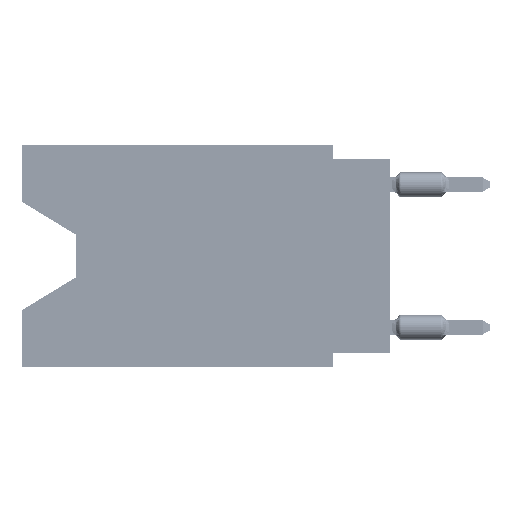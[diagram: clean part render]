
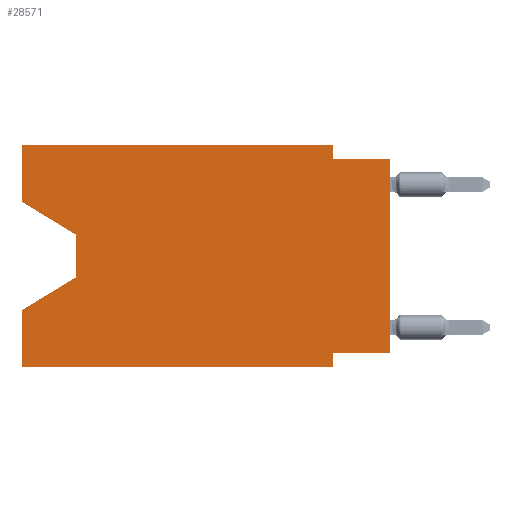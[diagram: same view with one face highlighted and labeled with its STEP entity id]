
A CAD part, left-side view. The second image highlights one B-rep face of the part: STEP entity #28571.
In plain terms, the highlighted planar face has unit normal (-1, 0, 0).
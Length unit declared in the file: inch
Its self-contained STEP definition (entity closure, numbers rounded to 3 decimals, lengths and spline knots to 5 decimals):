
#1226 = ORIENTED_EDGE ( 'NONE', *, *, #63937, .T. ) ;
#1732 = VERTEX_POINT ( 'NONE', #47006 ) ;
#1911 = AXIS2_PLACEMENT_3D ( 'NONE', #13726, #6431, #18738 ) ;
#3129 = ORIENTED_EDGE ( 'NONE', *, *, #56652, .T. ) ;
#3431 = DIRECTION ( 'NONE',  ( 0., 0., 1. ) ) ;
#3860 = VECTOR ( 'NONE', #61760, 39.37008 ) ;
#3981 = EDGE_CURVE ( 'NONE', #13742, #73121, #71780, .T. ) ;
#4955 = EDGE_LOOP ( 'NONE', ( #50636, #10048, #3129, #48341, #44960, #50207, #41376, #1226, #11884, #43274, #49702, #40008 ) ) ;
#5191 = LINE ( 'NONE', #29465, #14476 ) ;
#5551 = CARTESIAN_POINT ( 'NONE',  ( 0., 0., -0.025 ) ) ;
#6381 = VERTEX_POINT ( 'NONE', #11657 ) ;
#6431 = DIRECTION ( 'NONE',  ( 1., 0., 0. ) ) ;
#7757 = VECTOR ( 'NONE', #19069, 39.37008 ) ;
#9635 = VECTOR ( 'NONE', #69678, 39.37008 ) ;
#10048 = ORIENTED_EDGE ( 'NONE', *, *, #52039, .T. ) ;
#10237 = CARTESIAN_POINT ( 'NONE',  ( 0., 0.55, -0.158 ) ) ;
#10788 = CARTESIAN_POINT ( 'NONE',  ( 0., 0.55, -0.158 ) ) ;
#11657 = CARTESIAN_POINT ( 'NONE',  ( 0., 0., -0.365 ) ) ;
#11800 = CARTESIAN_POINT ( 'NONE',  ( 0., 0.1, -0.365 ) ) ;
#11804 = VECTOR ( 'NONE', #49444, 39.37008 ) ;
#11884 = ORIENTED_EDGE ( 'NONE', *, *, #3981, .F. ) ;
#11947 = VERTEX_POINT ( 'NONE', #71913 ) ;
#12646 = VERTEX_POINT ( 'NONE', #30132 ) ;
#13311 = EDGE_CURVE ( 'NONE', #67761, #75361, #25437, .T. ) ;
#13726 = CARTESIAN_POINT ( 'NONE',  ( 0., 0.645, 0. ) ) ;
#13742 = VERTEX_POINT ( 'NONE', #60339 ) ;
#13763 = VERTEX_POINT ( 'NONE', #42280 ) ;
#14257 = VECTOR ( 'NONE', #33912, 39.37008 ) ;
#14476 = VECTOR ( 'NONE', #34074, 39.37008 ) ;
#15251 = LINE ( 'NONE', #10237, #34022 ) ;
#15490 = EDGE_CURVE ( 'NONE', #12646, #13763, #5191, .T. ) ;
#18738 = DIRECTION ( 'NONE',  ( 0., 0., -1. ) ) ;
#19069 = DIRECTION ( 'NONE',  ( 0., -1., 0. ) ) ;
#19506 = PLANE ( 'NONE',  #1911 ) ;
#20638 = LINE ( 'NONE', #74440, #3860 ) ;
#21206 = DIRECTION ( 'NONE',  ( 0., 0., 1. ) ) ;
#21281 = EDGE_CURVE ( 'NONE', #63034, #13742, #20638, .T. ) ;
#24165 = VERTEX_POINT ( 'NONE', #71006 ) ;
#25437 = LINE ( 'NONE', #65808, #52499 ) ;
#27001 = LINE ( 'NONE', #73897, #65844 ) ;
#28571 = ADVANCED_FACE ( 'NONE', ( #66426 ), #19506, .F. ) ;
#29465 = CARTESIAN_POINT ( 'NONE',  ( 0., 0.645, -0.39 ) ) ;
#30132 = CARTESIAN_POINT ( 'NONE',  ( 0., 0.645, -0.39 ) ) ;
#30488 = EDGE_CURVE ( 'NONE', #12646, #11947, #27001, .T. ) ;
#30723 = CARTESIAN_POINT ( 'NONE',  ( 0., 0.1, -0.39 ) ) ;
#31454 = CARTESIAN_POINT ( 'NONE',  ( 0., 0.1, 0. ) ) ;
#33912 = DIRECTION ( 'NONE',  ( 0., -1., 0. ) ) ;
#34022 = VECTOR ( 'NONE', #74470, 39.37008 ) ;
#34074 = DIRECTION ( 'NONE',  ( 0., -1., 0. ) ) ;
#37645 = VERTEX_POINT ( 'NONE', #11800 ) ;
#37910 = LINE ( 'NONE', #43683, #57567 ) ;
#37973 = EDGE_CURVE ( 'NONE', #6381, #37645, #44080, .T. ) ;
#40008 = ORIENTED_EDGE ( 'NONE', *, *, #72026, .F. ) ;
#41376 = ORIENTED_EDGE ( 'NONE', *, *, #37973, .F. ) ;
#41501 = CARTESIAN_POINT ( 'NONE',  ( 0., 0.645, -0.10025 ) ) ;
#42280 = CARTESIAN_POINT ( 'NONE',  ( 0., 0.1, -0.39 ) ) ;
#43274 = ORIENTED_EDGE ( 'NONE', *, *, #21281, .F. ) ;
#43683 = CARTESIAN_POINT ( 'NONE',  ( 0., 0.55, -0.232 ) ) ;
#43889 = DIRECTION ( 'NONE',  ( 0., -0.855, -0.519 ) ) ;
#44080 = LINE ( 'NONE', #66743, #11804 ) ;
#44960 = ORIENTED_EDGE ( 'NONE', *, *, #15490, .T. ) ;
#46224 = LINE ( 'NONE', #70075, #9635 ) ;
#47006 = CARTESIAN_POINT ( 'NONE',  ( 0., 0.645, 0. ) ) ;
#47649 = LINE ( 'NONE', #30723, #67145 ) ;
#48341 = ORIENTED_EDGE ( 'NONE', *, *, #30488, .F. ) ;
#49444 = DIRECTION ( 'NONE',  ( 0., 1., 0. ) ) ;
#49702 = ORIENTED_EDGE ( 'NONE', *, *, #67223, .F. ) ;
#50207 = ORIENTED_EDGE ( 'NONE', *, *, #67865, .F. ) ;
#50387 = LINE ( 'NONE', #69209, #53221 ) ;
#50636 = ORIENTED_EDGE ( 'NONE', *, *, #13311, .T. ) ;
#51610 = LINE ( 'NONE', #55830, #14257 ) ;
#52039 = EDGE_CURVE ( 'NONE', #75361, #24165, #15251, .T. ) ;
#52499 = VECTOR ( 'NONE', #43889, 39.37008 ) ;
#53221 = VECTOR ( 'NONE', #3431, 39.37008 ) ;
#53394 = DIRECTION ( 'NONE',  ( 0., 0., -1. ) ) ;
#55830 = CARTESIAN_POINT ( 'NONE',  ( 0., 0.645, 0. ) ) ;
#56652 = EDGE_CURVE ( 'NONE', #24165, #11947, #37910, .T. ) ;
#57567 = VECTOR ( 'NONE', #72905, 39.37008 ) ;
#60242 = CARTESIAN_POINT ( 'NONE',  ( 0., 0., -0.025 ) ) ;
#60339 = CARTESIAN_POINT ( 'NONE',  ( 0., 0.1, -0.025 ) ) ;
#61760 = DIRECTION ( 'NONE',  ( 0., 0., -1. ) ) ;
#63034 = VERTEX_POINT ( 'NONE', #31454 ) ;
#63937 = EDGE_CURVE ( 'NONE', #6381, #73121, #50387, .T. ) ;
#65808 = CARTESIAN_POINT ( 'NONE',  ( 0., 0.645, -0.10025 ) ) ;
#65844 = VECTOR ( 'NONE', #21206, 39.37008 ) ;
#66426 = FACE_OUTER_BOUND ( 'NONE', #4955, .T. ) ;
#66743 = CARTESIAN_POINT ( 'NONE',  ( 0., 0., -0.365 ) ) ;
#67145 = VECTOR ( 'NONE', #53394, 39.37008 ) ;
#67223 = EDGE_CURVE ( 'NONE', #1732, #63034, #51610, .T. ) ;
#67761 = VERTEX_POINT ( 'NONE', #41501 ) ;
#67865 = EDGE_CURVE ( 'NONE', #37645, #13763, #47649, .T. ) ;
#69209 = CARTESIAN_POINT ( 'NONE',  ( 0., 0., 0. ) ) ;
#69678 = DIRECTION ( 'NONE',  ( 0., 0., 1. ) ) ;
#70075 = CARTESIAN_POINT ( 'NONE',  ( 0., 0.645, 0. ) ) ;
#71006 = CARTESIAN_POINT ( 'NONE',  ( 0., 0.55, -0.232 ) ) ;
#71780 = LINE ( 'NONE', #60242, #7757 ) ;
#71913 = CARTESIAN_POINT ( 'NONE',  ( 0., 0.645, -0.28975 ) ) ;
#72026 = EDGE_CURVE ( 'NONE', #67761, #1732, #46224, .T. ) ;
#72905 = DIRECTION ( 'NONE',  ( 0., 0.855, -0.519 ) ) ;
#73121 = VERTEX_POINT ( 'NONE', #5551 ) ;
#73897 = CARTESIAN_POINT ( 'NONE',  ( 0., 0.645, 0. ) ) ;
#74440 = CARTESIAN_POINT ( 'NONE',  ( 0., 0.1, 0. ) ) ;
#74470 = DIRECTION ( 'NONE',  ( 0., 0., -1. ) ) ;
#75361 = VERTEX_POINT ( 'NONE', #10788 ) ;
